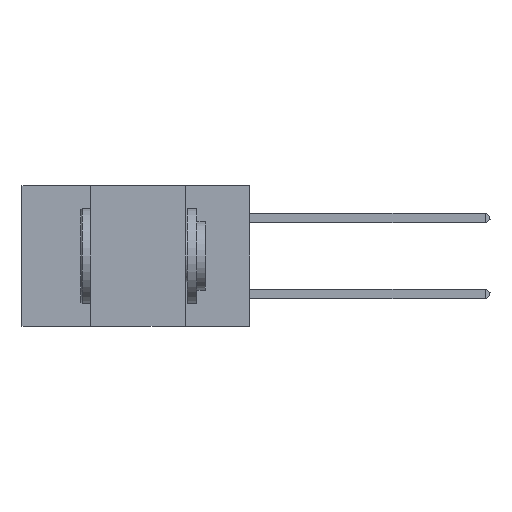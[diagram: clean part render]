
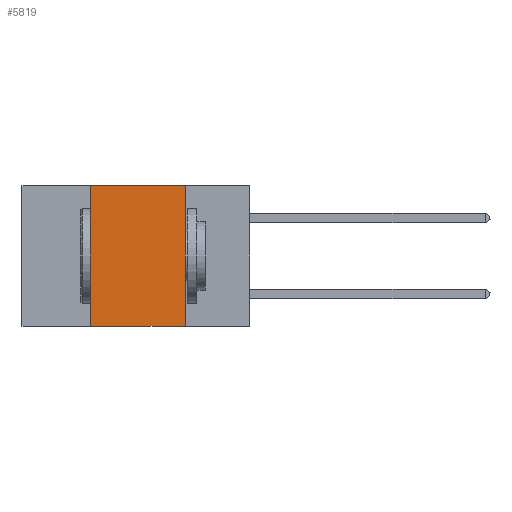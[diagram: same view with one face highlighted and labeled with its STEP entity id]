
A CAD part, left-side view. The second image highlights one B-rep face of the part: STEP entity #5819.
In plain terms, the highlighted planar face has unit normal (-1, 0, 0).
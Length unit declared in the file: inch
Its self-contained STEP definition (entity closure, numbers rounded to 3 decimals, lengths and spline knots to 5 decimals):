
#363 = DIRECTION ( 'NONE',  ( 0., -1., 0. ) ) ;
#420 = VERTEX_POINT ( 'NONE', #933 ) ;
#432 = CARTESIAN_POINT ( 'NONE',  ( 0., 0.6, 0. ) ) ;
#485 = LINE ( 'NONE', #2136, #5327 ) ;
#912 = VERTEX_POINT ( 'NONE', #6256 ) ;
#933 = CARTESIAN_POINT ( 'NONE',  ( 0., 0.42, 0. ) ) ;
#1034 = DIRECTION ( 'NONE',  ( 0., 0., 1. ) ) ;
#1429 = LINE ( 'NONE', #4938, #8989 ) ;
#2136 = CARTESIAN_POINT ( 'NONE',  ( 0., 0.42, 0. ) ) ;
#2482 = ORIENTED_EDGE ( 'NONE', *, *, #10774, .F. ) ;
#2872 = PLANE ( 'NONE',  #14380 ) ;
#3272 = EDGE_CURVE ( 'NONE', #11469, #912, #3903, .T. ) ;
#3667 = CARTESIAN_POINT ( 'NONE',  ( 0., 0.42, -0.37 ) ) ;
#3903 = LINE ( 'NONE', #7993, #12163 ) ;
#3937 = DIRECTION ( 'NONE',  ( 1., 0., 0. ) ) ;
#3986 = DIRECTION ( 'NONE',  ( 0., 0., -1. ) ) ;
#4704 = CARTESIAN_POINT ( 'NONE',  ( 0., 0.17, 0. ) ) ;
#4938 = CARTESIAN_POINT ( 'NONE',  ( 0., 0.6, 0. ) ) ;
#5019 = EDGE_CURVE ( 'NONE', #6761, #912, #11189, .T. ) ;
#5327 = VECTOR ( 'NONE', #1034, 39.37008 ) ;
#5601 = ORIENTED_EDGE ( 'NONE', *, *, #8900, .F. ) ;
#5819 = ADVANCED_FACE ( 'NONE', ( #8507 ), #2872, .F. ) ;
#6256 = CARTESIAN_POINT ( 'NONE',  ( 0., 0.17, -0.37 ) ) ;
#6761 = VERTEX_POINT ( 'NONE', #9202 ) ;
#7993 = CARTESIAN_POINT ( 'NONE',  ( 0., 0.6, -0.37 ) ) ;
#8140 = DIRECTION ( 'NONE',  ( 0., 0., -1. ) ) ;
#8507 = FACE_OUTER_BOUND ( 'NONE', #10622, .T. ) ;
#8900 = EDGE_CURVE ( 'NONE', #11469, #420, #485, .T. ) ;
#8989 = VECTOR ( 'NONE', #363, 39.37008 ) ;
#9202 = CARTESIAN_POINT ( 'NONE',  ( 0., 0.17, 0. ) ) ;
#10622 = EDGE_LOOP ( 'NONE', ( #11070, #2482, #5601, #10656 ) ) ;
#10656 = ORIENTED_EDGE ( 'NONE', *, *, #3272, .T. ) ;
#10774 = EDGE_CURVE ( 'NONE', #420, #6761, #1429, .T. ) ;
#10833 = VECTOR ( 'NONE', #8140, 39.37008 ) ;
#11070 = ORIENTED_EDGE ( 'NONE', *, *, #5019, .F. ) ;
#11189 = LINE ( 'NONE', #4704, #10833 ) ;
#11469 = VERTEX_POINT ( 'NONE', #3667 ) ;
#11587 = DIRECTION ( 'NONE',  ( 0., -1., 0. ) ) ;
#12163 = VECTOR ( 'NONE', #11587, 39.37008 ) ;
#14380 = AXIS2_PLACEMENT_3D ( 'NONE', #432, #3937, #3986 ) ;
